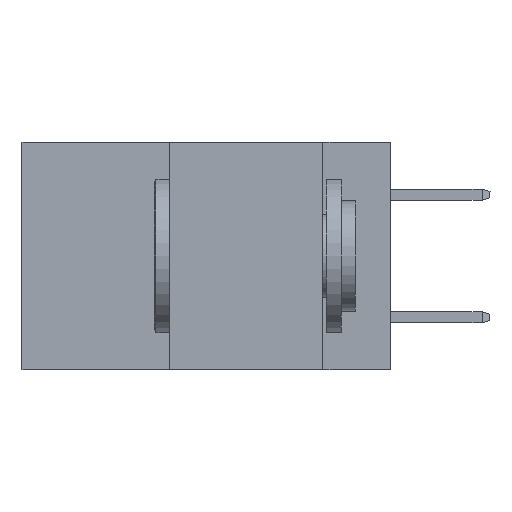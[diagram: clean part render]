
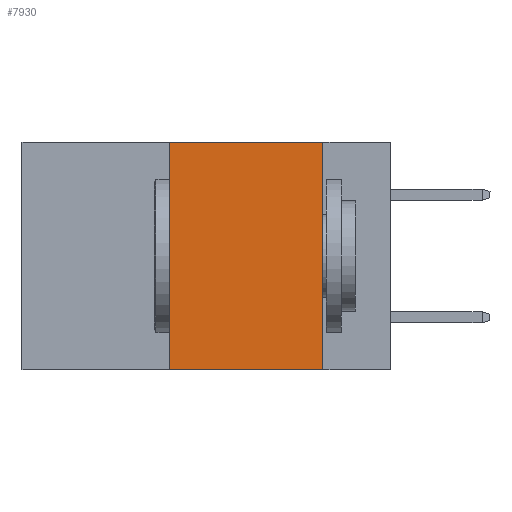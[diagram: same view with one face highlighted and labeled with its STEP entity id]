
A CAD part, left-side view. The second image highlights one B-rep face of the part: STEP entity #7930.
In plain terms, the highlighted planar face has unit normal (-1, 0, 0).
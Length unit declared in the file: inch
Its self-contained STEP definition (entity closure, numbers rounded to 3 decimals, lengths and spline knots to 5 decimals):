
#719 = EDGE_CURVE ( 'NONE', #12604, #8710, #10692, .T. ) ;
#1205 = EDGE_LOOP ( 'NONE', ( #4532, #5444, #12401, #3726 ) ) ;
#1423 = CARTESIAN_POINT ( 'NONE',  ( 0., 0.11, 0. ) ) ;
#2371 = VERTEX_POINT ( 'NONE', #12556 ) ;
#2476 = EDGE_CURVE ( 'NONE', #12604, #2371, #11507, .T. ) ;
#2762 = VECTOR ( 'NONE', #11959, 39.37008 ) ;
#2919 = DIRECTION ( 'NONE',  ( 0., 0., -1. ) ) ;
#3043 = CARTESIAN_POINT ( 'NONE',  ( 0., 0.11, 0. ) ) ;
#3465 = PLANE ( 'NONE',  #9823 ) ;
#3681 = EDGE_CURVE ( 'NONE', #8045, #2371, #10986, .T. ) ;
#3726 = ORIENTED_EDGE ( 'NONE', *, *, #2476, .T. ) ;
#4532 = ORIENTED_EDGE ( 'NONE', *, *, #3681, .F. ) ;
#4549 = DIRECTION ( 'NONE',  ( 1., 0., 0. ) ) ;
#4860 = DIRECTION ( 'NONE',  ( 0., -1., 0. ) ) ;
#5418 = CARTESIAN_POINT ( 'NONE',  ( 0., 0.6, -0.37 ) ) ;
#5444 = ORIENTED_EDGE ( 'NONE', *, *, #5659, .F. ) ;
#5659 = EDGE_CURVE ( 'NONE', #8710, #8045, #11095, .T. ) ;
#7612 = CARTESIAN_POINT ( 'NONE',  ( 0., 0.36, 0. ) ) ;
#7930 = ADVANCED_FACE ( 'NONE', ( #10878 ), #3465, .F. ) ;
#8045 = VERTEX_POINT ( 'NONE', #1423 ) ;
#8710 = VERTEX_POINT ( 'NONE', #13148 ) ;
#8730 = VECTOR ( 'NONE', #4860, 39.37008 ) ;
#8822 = VECTOR ( 'NONE', #12744, 39.37008 ) ;
#9823 = AXIS2_PLACEMENT_3D ( 'NONE', #10671, #4549, #11715 ) ;
#10671 = CARTESIAN_POINT ( 'NONE',  ( 0., 0.6, 0. ) ) ;
#10692 = LINE ( 'NONE', #7612, #2762 ) ;
#10878 = FACE_OUTER_BOUND ( 'NONE', #1205, .T. ) ;
#10986 = LINE ( 'NONE', #3043, #11315 ) ;
#11095 = LINE ( 'NONE', #12023, #8730 ) ;
#11315 = VECTOR ( 'NONE', #2919, 39.37008 ) ;
#11507 = LINE ( 'NONE', #5418, #8822 ) ;
#11715 = DIRECTION ( 'NONE',  ( 0., 0., -1. ) ) ;
#11738 = CARTESIAN_POINT ( 'NONE',  ( 0., 0.36, -0.37 ) ) ;
#11959 = DIRECTION ( 'NONE',  ( 0., 0., 1. ) ) ;
#12023 = CARTESIAN_POINT ( 'NONE',  ( 0., 0.6, 0. ) ) ;
#12401 = ORIENTED_EDGE ( 'NONE', *, *, #719, .F. ) ;
#12556 = CARTESIAN_POINT ( 'NONE',  ( 0., 0.11, -0.37 ) ) ;
#12604 = VERTEX_POINT ( 'NONE', #11738 ) ;
#12744 = DIRECTION ( 'NONE',  ( 0., -1., 0. ) ) ;
#13148 = CARTESIAN_POINT ( 'NONE',  ( 0., 0.36, 0. ) ) ;
